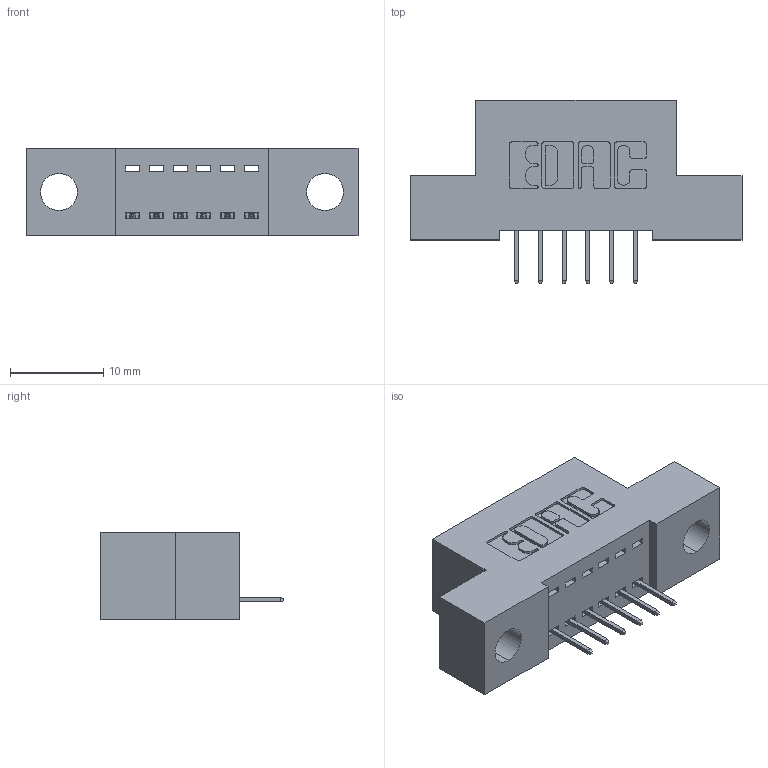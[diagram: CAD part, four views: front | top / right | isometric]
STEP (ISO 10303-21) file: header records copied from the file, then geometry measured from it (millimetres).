
FILE_DESCRIPTION (( 'STEP AP203' ), '1' );
FILE_NAME ('342-006-524-104.STEP', '2018-08-10T11:26:13', ( '' ), ( '' ), 'SwSTEP 2.0', 'SolidWorks 2016', '' );
FILE_SCHEMA (( 'CONFIG_CONTROL_DESIGN' ));
Length unit declared in the file: inch
Products named in the file (3): 342 Part_.156 TH; 345-292-001_345-293-124; 342-006-524-104
Assembly tree (7 placements, depth 2):
  342-006-524-104
    342 Part_.156 TH
    345-292-001_345-293-124  x6
Bounding box: 35.56 x 19.69 x 9.4 mm (x, y, z)
Volume: 2874.6 mm3; surface area: 3294.2 mm2
Topology: 7 solids, 7 shells, 482 faces, 1379 edges, 894 vertices
Faces by surface type: plane 354, cylinder 128
Entity records: 8269 total; most frequent: CARTESIAN_POINT 1436, ORIENTED_EDGE 1378, DIRECTION 1285, EDGE_CURVE 689, VECTOR 565, LINE 565, VERTEX_POINT 454, AXIS2_PLACEMENT_3D 360
